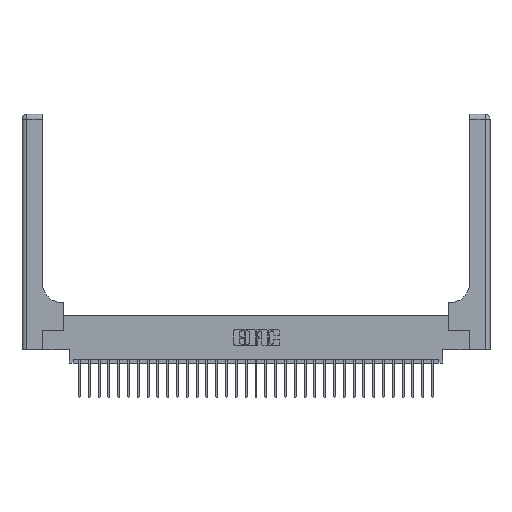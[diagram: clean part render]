
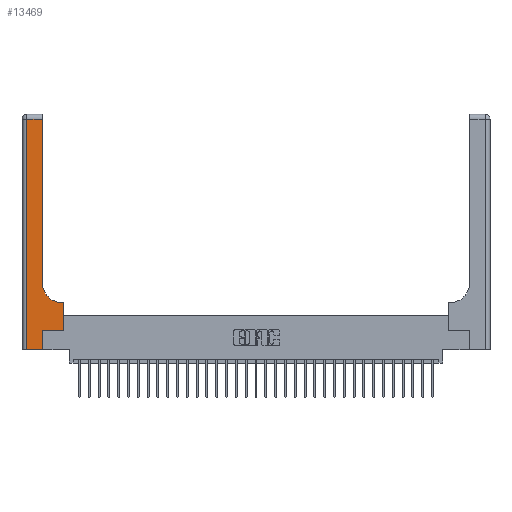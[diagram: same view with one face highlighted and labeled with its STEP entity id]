
A CAD part, top view. The second image highlights one B-rep face of the part: STEP entity #13469.
In plain terms, the highlighted planar face has unit normal (0, 0, 1).
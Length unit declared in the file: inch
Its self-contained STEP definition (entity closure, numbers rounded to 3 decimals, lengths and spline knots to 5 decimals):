
#196 = CARTESIAN_POINT ( 'NONE',  ( 0., 2.94, 0.37 ) ) ;
#335 = DIRECTION ( 'NONE',  ( 1., 0., 0. ) ) ;
#1484 = ORIENTED_EDGE ( 'NONE', *, *, #24336, .T. ) ;
#1584 = CARTESIAN_POINT ( 'NONE',  ( 0.265, 0.25, 0.37 ) ) ;
#1885 = EDGE_LOOP ( 'NONE', ( #25743, #14385, #13242, #6405, #21252, #18289, #1484, #28629, #17004 ) ) ;
#2372 = CARTESIAN_POINT ( 'NONE',  ( 0., 3., 0.37 ) ) ;
#2545 = DIRECTION ( 'NONE',  ( -1., 0., 0. ) ) ;
#3180 = EDGE_CURVE ( 'NONE', #18704, #7145, #28419, .T. ) ;
#3375 = VECTOR ( 'NONE', #14673, 39.37008 ) ;
#3454 = LINE ( 'NONE', #19714, #3687 ) ;
#3601 = DIRECTION ( 'NONE',  ( 0., 1., 0. ) ) ;
#3687 = VECTOR ( 'NONE', #3601, 39.37008 ) ;
#3816 = CARTESIAN_POINT ( 'NONE',  ( 0.26, 2.94, 0.37 ) ) ;
#3976 = EDGE_CURVE ( 'NONE', #22053, #22632, #8281, .T. ) ;
#4438 = DIRECTION ( 'NONE',  ( -1., 0., 0. ) ) ;
#5224 = CARTESIAN_POINT ( 'NONE',  ( 0.26, 3., 0.37 ) ) ;
#5353 = EDGE_CURVE ( 'NONE', #26860, #15721, #22915, .T. ) ;
#5669 = LINE ( 'NONE', #1584, #7482 ) ;
#6405 = ORIENTED_EDGE ( 'NONE', *, *, #13385, .T. ) ;
#6512 = EDGE_CURVE ( 'NONE', #22632, #9733, #5669, .T. ) ;
#7132 = VECTOR ( 'NONE', #13381, 39.37008 ) ;
#7145 = VERTEX_POINT ( 'NONE', #22824 ) ;
#7482 = VECTOR ( 'NONE', #29817, 39.37008 ) ;
#7818 = VECTOR ( 'NONE', #18506, 39.37008 ) ;
#8281 = LINE ( 'NONE', #17678, #18407 ) ;
#8334 = LINE ( 'NONE', #5224, #3375 ) ;
#9118 = CARTESIAN_POINT ( 'NONE',  ( 0., 0., 0.37 ) ) ;
#9733 = VERTEX_POINT ( 'NONE', #29584 ) ;
#10766 = CARTESIAN_POINT ( 'NONE',  ( 0.06, 3., 0.37 ) ) ;
#12197 = CARTESIAN_POINT ( 'NONE',  ( 0.26, 0.6, 0.37 ) ) ;
#12968 = VECTOR ( 'NONE', #2545, 39.37008 ) ;
#13242 = ORIENTED_EDGE ( 'NONE', *, *, #5353, .T. ) ;
#13381 = DIRECTION ( 'NONE',  ( 0., -1., 0. ) ) ;
#13385 = EDGE_CURVE ( 'NONE', #15721, #22053, #30587, .T. ) ;
#13469 = ADVANCED_FACE ( 'NONE', ( #25460 ), #16206, .F. ) ;
#14301 = CIRCLE ( 'NONE', #25124, 0.25 ) ;
#14326 = DIRECTION ( 'NONE',  ( 0., 0., -1. ) ) ;
#14385 = ORIENTED_EDGE ( 'NONE', *, *, #27222, .T. ) ;
#14673 = DIRECTION ( 'NONE',  ( 0., 1., 0. ) ) ;
#15721 = VERTEX_POINT ( 'NONE', #21125 ) ;
#16206 = PLANE ( 'NONE',  #27033 ) ;
#17004 = ORIENTED_EDGE ( 'NONE', *, *, #24152, .T. ) ;
#17139 = CARTESIAN_POINT ( 'NONE',  ( 0.26, 0.85, 0.37 ) ) ;
#17678 = CARTESIAN_POINT ( 'NONE',  ( 0.265, 0., 0.37 ) ) ;
#18289 = ORIENTED_EDGE ( 'NONE', *, *, #6512, .T. ) ;
#18407 = VECTOR ( 'NONE', #24774, 39.37008 ) ;
#18506 = DIRECTION ( 'NONE',  ( 1., 0., 0. ) ) ;
#18704 = VERTEX_POINT ( 'NONE', #24853 ) ;
#19132 = DIRECTION ( 'NONE',  ( -1., 0., 0. ) ) ;
#19714 = CARTESIAN_POINT ( 'NONE',  ( 0.528, 0.25, 0.37 ) ) ;
#20719 = CARTESIAN_POINT ( 'NONE',  ( 0.265, 0.25, 0.37 ) ) ;
#21125 = CARTESIAN_POINT ( 'NONE',  ( 0.06, 0., 0.37 ) ) ;
#21252 = ORIENTED_EDGE ( 'NONE', *, *, #3976, .T. ) ;
#21406 = LINE ( 'NONE', #196, #22886 ) ;
#22053 = VERTEX_POINT ( 'NONE', #27640 ) ;
#22632 = VERTEX_POINT ( 'NONE', #20719 ) ;
#22824 = CARTESIAN_POINT ( 'NONE',  ( 0.51, 0.6, 0.37 ) ) ;
#22886 = VECTOR ( 'NONE', #19132, 39.37008 ) ;
#22915 = LINE ( 'NONE', #10766, #7132 ) ;
#23462 = EDGE_CURVE ( 'NONE', #30317, #26840, #8334, .T. ) ;
#24152 = EDGE_CURVE ( 'NONE', #7145, #30317, #14301, .T. ) ;
#24336 = EDGE_CURVE ( 'NONE', #9733, #18704, #3454, .T. ) ;
#24774 = DIRECTION ( 'NONE',  ( 0., 1., 0. ) ) ;
#24853 = CARTESIAN_POINT ( 'NONE',  ( 0.528, 0.6, 0.37 ) ) ;
#25124 = AXIS2_PLACEMENT_3D ( 'NONE', #26066, #14326, #335 ) ;
#25460 = FACE_OUTER_BOUND ( 'NONE', #1885, .T. ) ;
#25627 = DIRECTION ( 'NONE',  ( 0., 0., -1. ) ) ;
#25743 = ORIENTED_EDGE ( 'NONE', *, *, #23462, .T. ) ;
#26066 = CARTESIAN_POINT ( 'NONE',  ( 0.51, 0.85, 0.37 ) ) ;
#26840 = VERTEX_POINT ( 'NONE', #3816 ) ;
#26860 = VERTEX_POINT ( 'NONE', #27328 ) ;
#27033 = AXIS2_PLACEMENT_3D ( 'NONE', #2372, #25627, #4438 ) ;
#27222 = EDGE_CURVE ( 'NONE', #26840, #26860, #21406, .T. ) ;
#27328 = CARTESIAN_POINT ( 'NONE',  ( 0.06, 2.94, 0.37 ) ) ;
#27640 = CARTESIAN_POINT ( 'NONE',  ( 0.265, 0., 0.37 ) ) ;
#28419 = LINE ( 'NONE', #12197, #12968 ) ;
#28629 = ORIENTED_EDGE ( 'NONE', *, *, #3180, .T. ) ;
#29584 = CARTESIAN_POINT ( 'NONE',  ( 0.528, 0.25, 0.37 ) ) ;
#29817 = DIRECTION ( 'NONE',  ( 1., 0., 0. ) ) ;
#30317 = VERTEX_POINT ( 'NONE', #17139 ) ;
#30587 = LINE ( 'NONE', #9118, #7818 ) ;
